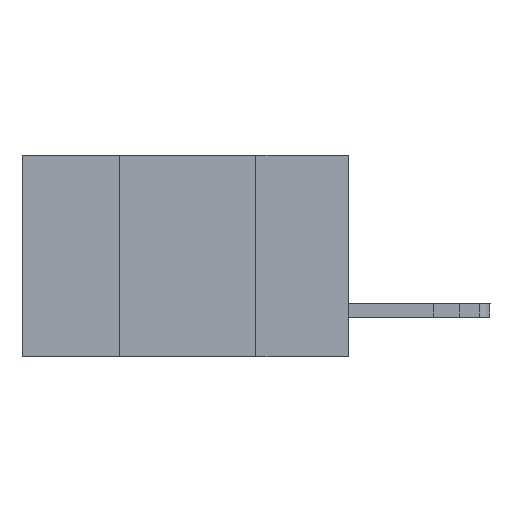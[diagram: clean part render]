
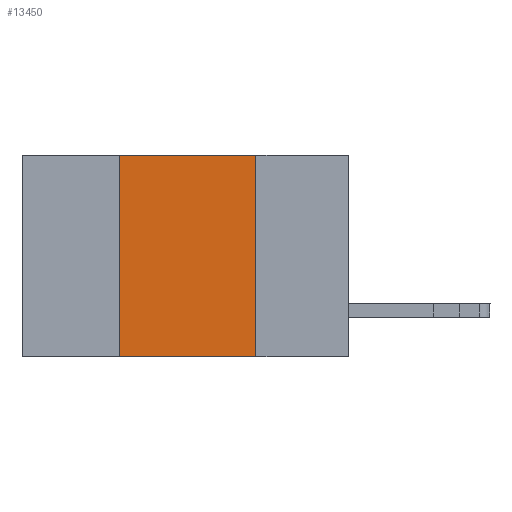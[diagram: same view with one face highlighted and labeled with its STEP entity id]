
A CAD part, left-side view. The second image highlights one B-rep face of the part: STEP entity #13450.
In plain terms, the highlighted planar face has unit normal (-1, 0, 0).
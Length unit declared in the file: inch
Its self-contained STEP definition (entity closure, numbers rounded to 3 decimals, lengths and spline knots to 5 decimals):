
#1519 = VERTEX_POINT ( 'NONE', #14073 ) ;
#1872 = LINE ( 'NONE', #10369, #10586 ) ;
#2806 = CARTESIAN_POINT ( 'NONE',  ( 0., 0.42, -0.37 ) ) ;
#2878 = VERTEX_POINT ( 'NONE', #9395 ) ;
#4195 = DIRECTION ( 'NONE',  ( 0., 0., 1. ) ) ;
#4272 = VECTOR ( 'NONE', #4195, 39.37008 ) ;
#4727 = DIRECTION ( 'NONE',  ( 0., -1., 0. ) ) ;
#4829 = PLANE ( 'NONE',  #15324 ) ;
#4909 = DIRECTION ( 'NONE',  ( 0., 0., -1. ) ) ;
#4947 = EDGE_CURVE ( 'NONE', #10740, #1519, #1872, .T. ) ;
#5207 = LINE ( 'NONE', #7411, #6577 ) ;
#5587 = EDGE_LOOP ( 'NONE', ( #11352, #6904, #14751, #9293 ) ) ;
#5651 = CARTESIAN_POINT ( 'NONE',  ( 0., 0.42, 0. ) ) ;
#5845 = CARTESIAN_POINT ( 'NONE',  ( 0., 0.6, 0. ) ) ;
#6158 = EDGE_CURVE ( 'NONE', #2878, #1519, #5207, .T. ) ;
#6577 = VECTOR ( 'NONE', #11227, 39.37008 ) ;
#6904 = ORIENTED_EDGE ( 'NONE', *, *, #12608, .F. ) ;
#6935 = CARTESIAN_POINT ( 'NONE',  ( 0., 0.6, 0. ) ) ;
#7411 = CARTESIAN_POINT ( 'NONE',  ( 0., 0.6, -0.37 ) ) ;
#7629 = LINE ( 'NONE', #2806, #4272 ) ;
#9062 = VERTEX_POINT ( 'NONE', #5651 ) ;
#9293 = ORIENTED_EDGE ( 'NONE', *, *, #6158, .T. ) ;
#9395 = CARTESIAN_POINT ( 'NONE',  ( 0., 0.42, -0.37 ) ) ;
#9760 = FACE_OUTER_BOUND ( 'NONE', #5587, .T. ) ;
#10334 = CARTESIAN_POINT ( 'NONE',  ( 0., 0.17, 0. ) ) ;
#10369 = CARTESIAN_POINT ( 'NONE',  ( 0., 0.17, -0.37 ) ) ;
#10389 = EDGE_CURVE ( 'NONE', #2878, #9062, #7629, .T. ) ;
#10586 = VECTOR ( 'NONE', #12702, 39.37008 ) ;
#10740 = VERTEX_POINT ( 'NONE', #10334 ) ;
#11227 = DIRECTION ( 'NONE',  ( 0., -1., 0. ) ) ;
#11352 = ORIENTED_EDGE ( 'NONE', *, *, #4947, .F. ) ;
#12608 = EDGE_CURVE ( 'NONE', #9062, #10740, #14178, .T. ) ;
#12702 = DIRECTION ( 'NONE',  ( 0., 0., -1. ) ) ;
#12766 = VECTOR ( 'NONE', #4727, 39.37008 ) ;
#13450 = ADVANCED_FACE ( 'NONE', ( #9760 ), #4829, .F. ) ;
#14073 = CARTESIAN_POINT ( 'NONE',  ( 0., 0.17, -0.37 ) ) ;
#14178 = LINE ( 'NONE', #6935, #12766 ) ;
#14751 = ORIENTED_EDGE ( 'NONE', *, *, #10389, .F. ) ;
#15324 = AXIS2_PLACEMENT_3D ( 'NONE', #5845, #15366, #4909 ) ;
#15366 = DIRECTION ( 'NONE',  ( 1., 0., 0. ) ) ;
